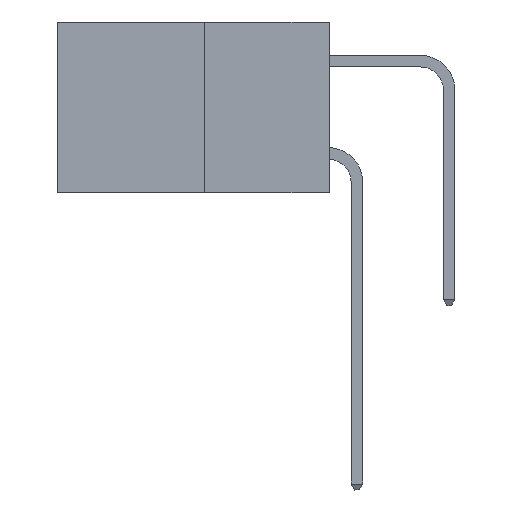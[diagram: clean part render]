
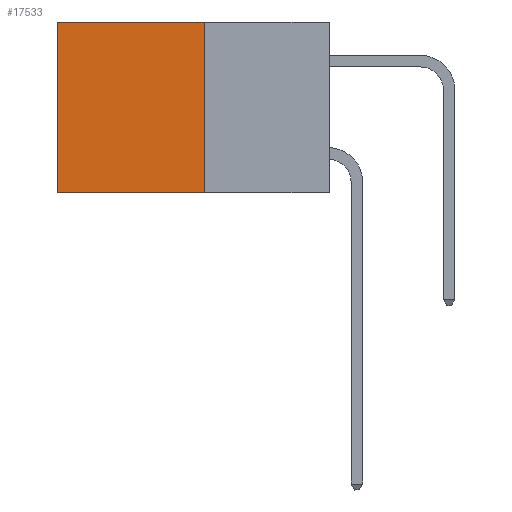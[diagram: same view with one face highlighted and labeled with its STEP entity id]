
A CAD part, left-side view. The second image highlights one B-rep face of the part: STEP entity #17533.
In plain terms, the highlighted planar face has unit normal (-1, 0, 0).
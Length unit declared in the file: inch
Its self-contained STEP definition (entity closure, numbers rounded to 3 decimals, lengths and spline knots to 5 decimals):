
#1840 = LINE ( 'NONE', #20039, #8237 ) ;
#2268 = EDGE_CURVE ( 'NONE', #17946, #5301, #17595, .T. ) ;
#2520 = VECTOR ( 'NONE', #7746, 39.37008 ) ;
#3742 = DIRECTION ( 'NONE',  ( 0., 0., -1. ) ) ;
#3801 = DIRECTION ( 'NONE',  ( 0., 0., -1. ) ) ;
#5301 = VERTEX_POINT ( 'NONE', #30773 ) ;
#6855 = EDGE_CURVE ( 'NONE', #26278, #9036, #14661, .T. ) ;
#7711 = EDGE_CURVE ( 'NONE', #26278, #17946, #1840, .T. ) ;
#7746 = DIRECTION ( 'NONE',  ( 0., 0., -1. ) ) ;
#8237 = VECTOR ( 'NONE', #3742, 39.37008 ) ;
#8901 = LINE ( 'NONE', #24035, #2520 ) ;
#9036 = VERTEX_POINT ( 'NONE', #23095 ) ;
#11884 = PLANE ( 'NONE',  #31538 ) ;
#14033 = CARTESIAN_POINT ( 'NONE',  ( 0.277, 0.27, 0. ) ) ;
#14121 = FACE_OUTER_BOUND ( 'NONE', #19627, .T. ) ;
#14661 = LINE ( 'NONE', #14033, #21929 ) ;
#14775 = ORIENTED_EDGE ( 'NONE', *, *, #2268, .F. ) ;
#17533 = ADVANCED_FACE ( 'NONE', ( #14121 ), #11884, .F. ) ;
#17595 = LINE ( 'NONE', #26739, #24020 ) ;
#17946 = VERTEX_POINT ( 'NONE', #29649 ) ;
#19036 = EDGE_CURVE ( 'NONE', #9036, #5301, #8901, .T. ) ;
#19627 = EDGE_LOOP ( 'NONE', ( #26779, #14775, #34819, #22273 ) ) ;
#20039 = CARTESIAN_POINT ( 'NONE',  ( 0.277, 0.27, -0.37 ) ) ;
#20107 = DIRECTION ( 'NONE',  ( 1., 0., 0. ) ) ;
#21929 = VECTOR ( 'NONE', #32922, 39.37008 ) ;
#22273 = ORIENTED_EDGE ( 'NONE', *, *, #6855, .T. ) ;
#22742 = CARTESIAN_POINT ( 'NONE',  ( 0.277, 0.27, -0.37 ) ) ;
#23095 = CARTESIAN_POINT ( 'NONE',  ( 0.277, 0.59, 0. ) ) ;
#24020 = VECTOR ( 'NONE', #25596, 39.37008 ) ;
#24035 = CARTESIAN_POINT ( 'NONE',  ( 0.277, 0.59, -0.37 ) ) ;
#25596 = DIRECTION ( 'NONE',  ( 0., 1., 0. ) ) ;
#26278 = VERTEX_POINT ( 'NONE', #34899 ) ;
#26739 = CARTESIAN_POINT ( 'NONE',  ( 0.277, 0.27, -0.37 ) ) ;
#26779 = ORIENTED_EDGE ( 'NONE', *, *, #19036, .T. ) ;
#29649 = CARTESIAN_POINT ( 'NONE',  ( 0.277, 0.27, -0.37 ) ) ;
#30773 = CARTESIAN_POINT ( 'NONE',  ( 0.277, 0.59, -0.37 ) ) ;
#31538 = AXIS2_PLACEMENT_3D ( 'NONE', #22742, #20107, #3801 ) ;
#32922 = DIRECTION ( 'NONE',  ( 0., 1., 0. ) ) ;
#34819 = ORIENTED_EDGE ( 'NONE', *, *, #7711, .F. ) ;
#34899 = CARTESIAN_POINT ( 'NONE',  ( 0.277, 0.27, 0. ) ) ;
